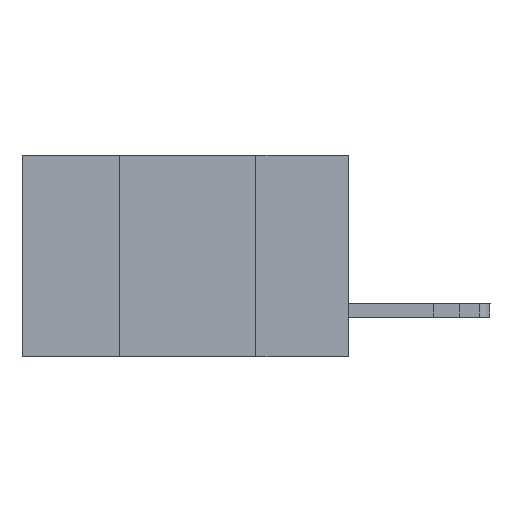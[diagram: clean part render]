
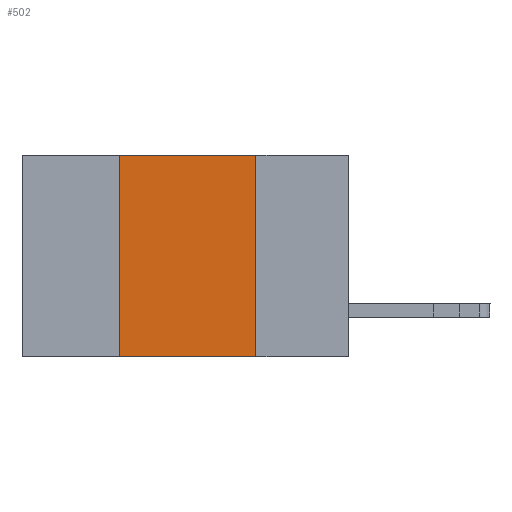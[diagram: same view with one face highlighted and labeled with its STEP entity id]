
A CAD part, left-side view. The second image highlights one B-rep face of the part: STEP entity #502.
In plain terms, the highlighted planar face has unit normal (-1, 0, 0).
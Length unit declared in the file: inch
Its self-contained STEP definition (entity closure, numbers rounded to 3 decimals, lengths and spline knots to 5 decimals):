
#224 = CARTESIAN_POINT ( 'NONE',  ( 0., 0.6, -0.37 ) ) ;
#387 = PLANE ( 'NONE',  #1776 ) ;
#434 = DIRECTION ( 'NONE',  ( 0., -1., 0. ) ) ;
#502 = ADVANCED_FACE ( 'NONE', ( #11230 ), #387, .F. ) ;
#557 = VECTOR ( 'NONE', #434, 39.37008 ) ;
#756 = CARTESIAN_POINT ( 'NONE',  ( 0., 0.17, 0. ) ) ;
#1309 = CARTESIAN_POINT ( 'NONE',  ( 0., 0.6, 0. ) ) ;
#1345 = VECTOR ( 'NONE', #6257, 39.37008 ) ;
#1767 = EDGE_LOOP ( 'NONE', ( #5353, #7551, #8230, #7195 ) ) ;
#1776 = AXIS2_PLACEMENT_3D ( 'NONE', #9408, #10063, #1980 ) ;
#1980 = DIRECTION ( 'NONE',  ( 0., 0., -1. ) ) ;
#2250 = EDGE_CURVE ( 'NONE', #8338, #6125, #3041, .T. ) ;
#2851 = EDGE_CURVE ( 'NONE', #8911, #8338, #9968, .T. ) ;
#3041 = LINE ( 'NONE', #1309, #557 ) ;
#3821 = VERTEX_POINT ( 'NONE', #4323 ) ;
#3840 = DIRECTION ( 'NONE',  ( 0., -1., 0. ) ) ;
#4038 = LINE ( 'NONE', #756, #5786 ) ;
#4323 = CARTESIAN_POINT ( 'NONE',  ( 0., 0.17, -0.37 ) ) ;
#4478 = CARTESIAN_POINT ( 'NONE',  ( 0., 0.17, 0. ) ) ;
#5353 = ORIENTED_EDGE ( 'NONE', *, *, #7295, .F. ) ;
#5438 = VECTOR ( 'NONE', #3840, 39.37008 ) ;
#5786 = VECTOR ( 'NONE', #9389, 39.37008 ) ;
#6125 = VERTEX_POINT ( 'NONE', #4478 ) ;
#6257 = DIRECTION ( 'NONE',  ( 0., 0., 1. ) ) ;
#6317 = CARTESIAN_POINT ( 'NONE',  ( 0., 0.42, 0. ) ) ;
#6541 = CARTESIAN_POINT ( 'NONE',  ( 0., 0.42, 0. ) ) ;
#6640 = CARTESIAN_POINT ( 'NONE',  ( 0., 0.42, -0.37 ) ) ;
#7195 = ORIENTED_EDGE ( 'NONE', *, *, #8357, .T. ) ;
#7295 = EDGE_CURVE ( 'NONE', #6125, #3821, #4038, .T. ) ;
#7551 = ORIENTED_EDGE ( 'NONE', *, *, #2250, .F. ) ;
#8230 = ORIENTED_EDGE ( 'NONE', *, *, #2851, .F. ) ;
#8298 = LINE ( 'NONE', #224, #5438 ) ;
#8338 = VERTEX_POINT ( 'NONE', #6541 ) ;
#8357 = EDGE_CURVE ( 'NONE', #8911, #3821, #8298, .T. ) ;
#8911 = VERTEX_POINT ( 'NONE', #6640 ) ;
#9389 = DIRECTION ( 'NONE',  ( 0., 0., -1. ) ) ;
#9408 = CARTESIAN_POINT ( 'NONE',  ( 0., 0.6, 0. ) ) ;
#9968 = LINE ( 'NONE', #6317, #1345 ) ;
#10063 = DIRECTION ( 'NONE',  ( 1., 0., 0. ) ) ;
#11230 = FACE_OUTER_BOUND ( 'NONE', #1767, .T. ) ;
